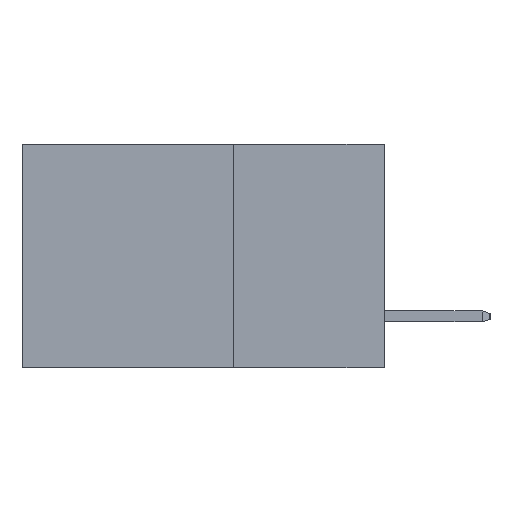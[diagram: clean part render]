
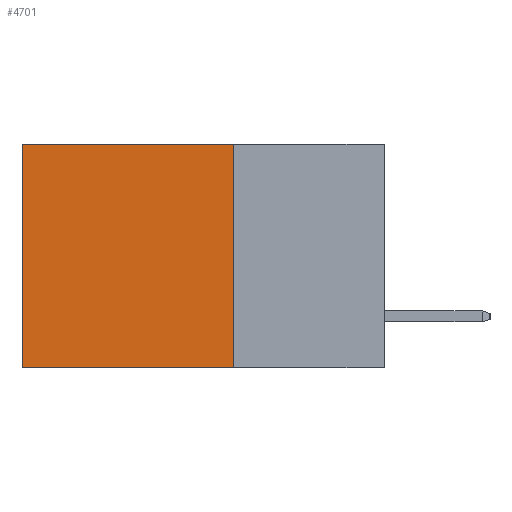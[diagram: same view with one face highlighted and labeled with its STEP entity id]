
A CAD part, left-side view. The second image highlights one B-rep face of the part: STEP entity #4701.
In plain terms, the highlighted planar face has unit normal (-1, 0, 0).
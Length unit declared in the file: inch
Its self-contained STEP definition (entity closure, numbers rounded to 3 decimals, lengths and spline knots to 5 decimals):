
#220 = ORIENTED_EDGE ( 'NONE', *, *, #13215, .F. ) ;
#1159 = CARTESIAN_POINT ( 'NONE',  ( 0.298, 0.25, 0. ) ) ;
#1373 = CARTESIAN_POINT ( 'NONE',  ( 0.298, 0.6, -0.37 ) ) ;
#1671 = CARTESIAN_POINT ( 'NONE',  ( 0.298, 0.25, 0. ) ) ;
#2411 = FACE_OUTER_BOUND ( 'NONE', #3502, .T. ) ;
#3175 = CARTESIAN_POINT ( 'NONE',  ( 0.298, 0.6, 0. ) ) ;
#3333 = EDGE_CURVE ( 'NONE', #6041, #6330, #8513, .T. ) ;
#3502 = EDGE_LOOP ( 'NONE', ( #7364, #220, #10872, #6273 ) ) ;
#3698 = VERTEX_POINT ( 'NONE', #4947 ) ;
#4380 = DIRECTION ( 'NONE',  ( 0., 1., 0. ) ) ;
#4701 = ADVANCED_FACE ( 'NONE', ( #2411 ), #10632, .F. ) ;
#4730 = CARTESIAN_POINT ( 'NONE',  ( 0.298, 0.25, -0.37 ) ) ;
#4947 = CARTESIAN_POINT ( 'NONE',  ( 0.298, 0.25, 0. ) ) ;
#5133 = VECTOR ( 'NONE', #4380, 39.37008 ) ;
#5143 = AXIS2_PLACEMENT_3D ( 'NONE', #5488, #9613, #6165 ) ;
#5150 = EDGE_CURVE ( 'NONE', #3698, #9180, #13733, .T. ) ;
#5488 = CARTESIAN_POINT ( 'NONE',  ( 0.298, 0.25, 0. ) ) ;
#5757 = VECTOR ( 'NONE', #8104, 39.37008 ) ;
#6041 = VERTEX_POINT ( 'NONE', #7242 ) ;
#6165 = DIRECTION ( 'NONE',  ( 0., 0., -1. ) ) ;
#6273 = ORIENTED_EDGE ( 'NONE', *, *, #10268, .T. ) ;
#6330 = VERTEX_POINT ( 'NONE', #1373 ) ;
#6881 = DIRECTION ( 'NONE',  ( 0., 0., -1. ) ) ;
#7242 = CARTESIAN_POINT ( 'NONE',  ( 0.298, 0.6, 0. ) ) ;
#7364 = ORIENTED_EDGE ( 'NONE', *, *, #3333, .T. ) ;
#8104 = DIRECTION ( 'NONE',  ( 0., 1., 0. ) ) ;
#8513 = LINE ( 'NONE', #3175, #11423 ) ;
#8518 = VECTOR ( 'NONE', #6881, 39.37008 ) ;
#9180 = VERTEX_POINT ( 'NONE', #4730 ) ;
#9613 = DIRECTION ( 'NONE',  ( 1., 0., 0. ) ) ;
#10268 = EDGE_CURVE ( 'NONE', #3698, #6041, #13962, .T. ) ;
#10632 = PLANE ( 'NONE',  #5143 ) ;
#10872 = ORIENTED_EDGE ( 'NONE', *, *, #5150, .F. ) ;
#11423 = VECTOR ( 'NONE', #13121, 39.37008 ) ;
#12232 = CARTESIAN_POINT ( 'NONE',  ( 0.298, 0.25, -0.37 ) ) ;
#13121 = DIRECTION ( 'NONE',  ( 0., 0., -1. ) ) ;
#13215 = EDGE_CURVE ( 'NONE', #9180, #6330, #14052, .T. ) ;
#13733 = LINE ( 'NONE', #1671, #8518 ) ;
#13962 = LINE ( 'NONE', #1159, #5757 ) ;
#14052 = LINE ( 'NONE', #12232, #5133 ) ;
